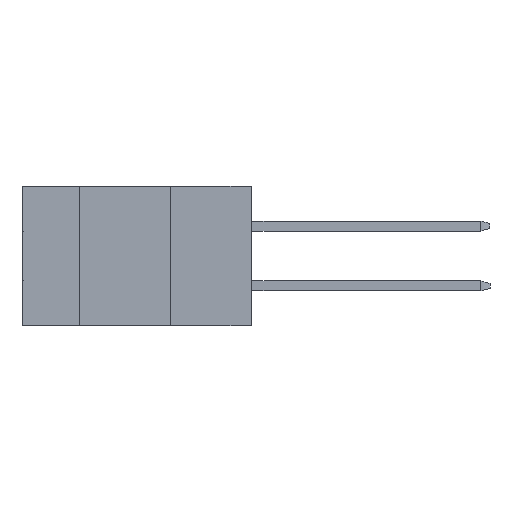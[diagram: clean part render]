
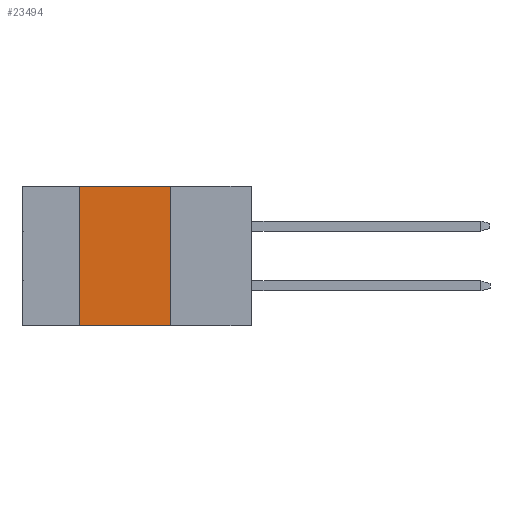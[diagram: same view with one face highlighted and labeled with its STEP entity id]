
A CAD part, left-side view. The second image highlights one B-rep face of the part: STEP entity #23494.
In plain terms, the highlighted planar face has unit normal (-1, 0, 0).
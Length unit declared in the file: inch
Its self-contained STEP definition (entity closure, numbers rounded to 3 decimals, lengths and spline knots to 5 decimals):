
#310 = PLANE ( 'NONE',  #14404 ) ;
#536 = ORIENTED_EDGE ( 'NONE', *, *, #14049, .F. ) ;
#697 = VERTEX_POINT ( 'NONE', #12531 ) ;
#939 = CARTESIAN_POINT ( 'NONE',  ( 0., 0.54, -0.437 ) ) ;
#1923 = ORIENTED_EDGE ( 'NONE', *, *, #10731, .F. ) ;
#3417 = LINE ( 'NONE', #10829, #12225 ) ;
#3665 = ORIENTED_EDGE ( 'NONE', *, *, #6788, .F. ) ;
#3803 = EDGE_LOOP ( 'NONE', ( #3665, #536, #1923, #12209 ) ) ;
#4312 = DIRECTION ( 'NONE',  ( 1., 0., 0. ) ) ;
#4561 = CARTESIAN_POINT ( 'NONE',  ( 0., 0.254, -0.437 ) ) ;
#5384 = VECTOR ( 'NONE', #19481, 39.37008 ) ;
#5559 = CARTESIAN_POINT ( 'NONE',  ( 0., 0.54, -0.437 ) ) ;
#6721 = DIRECTION ( 'NONE',  ( 0., -1., 0. ) ) ;
#6788 = EDGE_CURVE ( 'NONE', #8348, #7264, #13766, .T. ) ;
#6831 = CARTESIAN_POINT ( 'NONE',  ( 0., 0.72, 0. ) ) ;
#7264 = VERTEX_POINT ( 'NONE', #8874 ) ;
#7953 = FACE_OUTER_BOUND ( 'NONE', #3803, .T. ) ;
#8348 = VERTEX_POINT ( 'NONE', #16294 ) ;
#8874 = CARTESIAN_POINT ( 'NONE',  ( 0., 0.254, -0.437 ) ) ;
#9012 = DIRECTION ( 'NONE',  ( 0., -1., 0. ) ) ;
#10731 = EDGE_CURVE ( 'NONE', #17471, #697, #12950, .T. ) ;
#10829 = CARTESIAN_POINT ( 'NONE',  ( 0., 0.72, -0.437 ) ) ;
#11550 = EDGE_CURVE ( 'NONE', #17471, #7264, #3417, .T. ) ;
#12209 = ORIENTED_EDGE ( 'NONE', *, *, #11550, .T. ) ;
#12225 = VECTOR ( 'NONE', #9012, 39.37008 ) ;
#12531 = CARTESIAN_POINT ( 'NONE',  ( 0., 0.54, 0. ) ) ;
#12765 = LINE ( 'NONE', #6831, #23497 ) ;
#12950 = LINE ( 'NONE', #5559, #17114 ) ;
#13766 = LINE ( 'NONE', #4561, #5384 ) ;
#14049 = EDGE_CURVE ( 'NONE', #697, #8348, #12765, .T. ) ;
#14404 = AXIS2_PLACEMENT_3D ( 'NONE', #15574, #4312, #22969 ) ;
#15574 = CARTESIAN_POINT ( 'NONE',  ( 0., 0.72, 0. ) ) ;
#16294 = CARTESIAN_POINT ( 'NONE',  ( 0., 0.254, 0. ) ) ;
#16821 = DIRECTION ( 'NONE',  ( 0., 0., 1. ) ) ;
#17114 = VECTOR ( 'NONE', #16821, 39.37008 ) ;
#17471 = VERTEX_POINT ( 'NONE', #939 ) ;
#19481 = DIRECTION ( 'NONE',  ( 0., 0., -1. ) ) ;
#22969 = DIRECTION ( 'NONE',  ( 0., 0., -1. ) ) ;
#23494 = ADVANCED_FACE ( 'NONE', ( #7953 ), #310, .F. ) ;
#23497 = VECTOR ( 'NONE', #6721, 39.37008 ) ;
